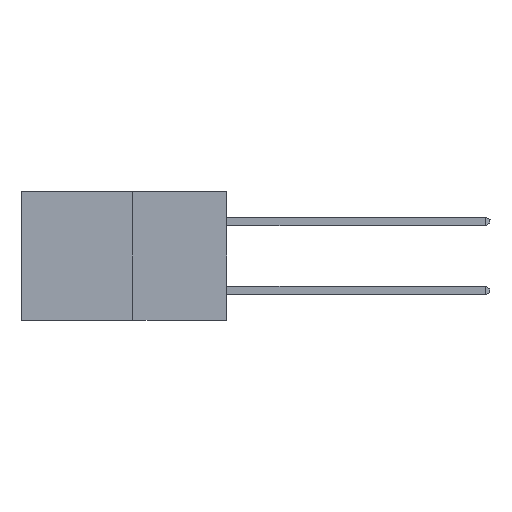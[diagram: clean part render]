
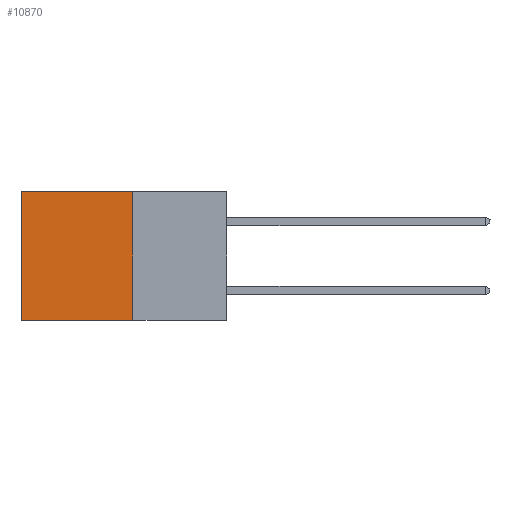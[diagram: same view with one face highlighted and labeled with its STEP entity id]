
A CAD part, left-side view. The second image highlights one B-rep face of the part: STEP entity #10870.
In plain terms, the highlighted planar face has unit normal (-1, 0, 0).
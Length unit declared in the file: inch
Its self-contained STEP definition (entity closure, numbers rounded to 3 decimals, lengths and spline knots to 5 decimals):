
#492 = CARTESIAN_POINT ( 'NONE',  ( 0.277, 0.59, 0. ) ) ;
#653 = DIRECTION ( 'NONE',  ( 1., 0., 0. ) ) ;
#1841 = CARTESIAN_POINT ( 'NONE',  ( 0.277, 0.27, 0. ) ) ;
#2334 = ORIENTED_EDGE ( 'NONE', *, *, #6799, .T. ) ;
#3001 = VECTOR ( 'NONE', #16839, 39.37008 ) ;
#3056 = DIRECTION ( 'NONE',  ( 0., 1., 0. ) ) ;
#3430 = CARTESIAN_POINT ( 'NONE',  ( 0.277, 0.27, -0.37 ) ) ;
#4324 = VERTEX_POINT ( 'NONE', #492 ) ;
#4492 = EDGE_CURVE ( 'NONE', #17642, #10776, #18636, .T. ) ;
#4639 = CARTESIAN_POINT ( 'NONE',  ( 0.277, 0.59, -0.37 ) ) ;
#5003 = LINE ( 'NONE', #9030, #5945 ) ;
#5045 = CARTESIAN_POINT ( 'NONE',  ( 0.277, 0.59, -0.37 ) ) ;
#5081 = CARTESIAN_POINT ( 'NONE',  ( 0.277, 0.27, -0.37 ) ) ;
#5931 = VERTEX_POINT ( 'NONE', #4639 ) ;
#5945 = VECTOR ( 'NONE', #3056, 39.37008 ) ;
#6566 = DIRECTION ( 'NONE',  ( 0., 0., -1. ) ) ;
#6799 = EDGE_CURVE ( 'NONE', #4324, #5931, #18546, .T. ) ;
#7650 = ORIENTED_EDGE ( 'NONE', *, *, #4492, .F. ) ;
#7796 = EDGE_LOOP ( 'NONE', ( #2334, #18053, #7650, #11655 ) ) ;
#9030 = CARTESIAN_POINT ( 'NONE',  ( 0.277, 0.27, 0. ) ) ;
#9453 = CARTESIAN_POINT ( 'NONE',  ( 0.277, 0.27, -0.37 ) ) ;
#9819 = VECTOR ( 'NONE', #6566, 39.37008 ) ;
#10776 = VERTEX_POINT ( 'NONE', #3430 ) ;
#10870 = ADVANCED_FACE ( 'NONE', ( #15854 ), #14061, .F. ) ;
#10930 = LINE ( 'NONE', #9453, #3001 ) ;
#11119 = DIRECTION ( 'NONE',  ( 0., 0., -1. ) ) ;
#11655 = ORIENTED_EDGE ( 'NONE', *, *, #13291, .T. ) ;
#11754 = AXIS2_PLACEMENT_3D ( 'NONE', #5081, #653, #11119 ) ;
#13291 = EDGE_CURVE ( 'NONE', #17642, #4324, #5003, .T. ) ;
#14061 = PLANE ( 'NONE',  #11754 ) ;
#14803 = VECTOR ( 'NONE', #16937, 39.37008 ) ;
#15854 = FACE_OUTER_BOUND ( 'NONE', #7796, .T. ) ;
#16813 = CARTESIAN_POINT ( 'NONE',  ( 0.277, 0.27, -0.37 ) ) ;
#16839 = DIRECTION ( 'NONE',  ( 0., 1., 0. ) ) ;
#16937 = DIRECTION ( 'NONE',  ( 0., 0., -1. ) ) ;
#17642 = VERTEX_POINT ( 'NONE', #1841 ) ;
#17704 = EDGE_CURVE ( 'NONE', #10776, #5931, #10930, .T. ) ;
#18053 = ORIENTED_EDGE ( 'NONE', *, *, #17704, .F. ) ;
#18546 = LINE ( 'NONE', #5045, #9819 ) ;
#18636 = LINE ( 'NONE', #16813, #14803 ) ;
